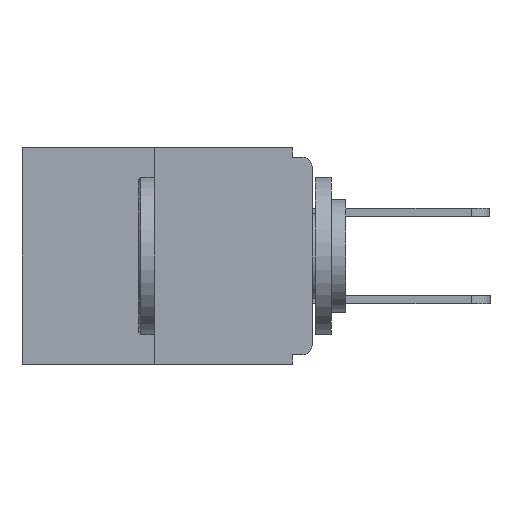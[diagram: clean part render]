
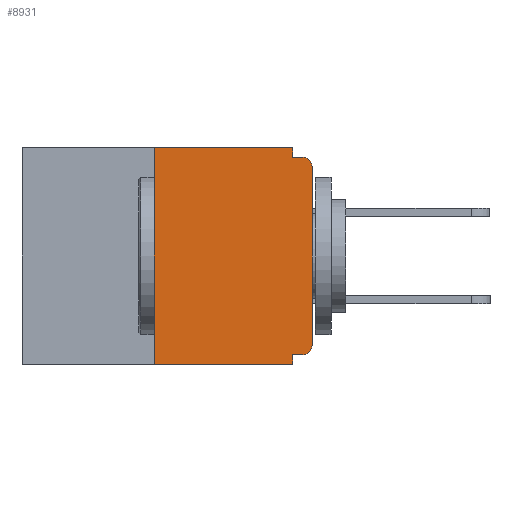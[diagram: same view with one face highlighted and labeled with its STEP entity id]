
A CAD part, left-side view. The second image highlights one B-rep face of the part: STEP entity #8931.
In plain terms, the highlighted planar face has unit normal (-1, 0, 0).
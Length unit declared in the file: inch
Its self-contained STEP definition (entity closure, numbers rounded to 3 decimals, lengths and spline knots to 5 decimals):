
#294 = VECTOR ( 'NONE', #5485, 39.37008 ) ;
#448 = AXIS2_PLACEMENT_3D ( 'NONE', #3779, #9084, #16150 ) ;
#1070 = CARTESIAN_POINT ( 'NONE',  ( 0., 0.031, -0.015 ) ) ;
#1130 = VERTEX_POINT ( 'NONE', #19791 ) ;
#1326 = CARTESIAN_POINT ( 'NONE',  ( 0., 0., -0.328 ) ) ;
#1334 = PLANE ( 'NONE',  #12542 ) ;
#1632 = CARTESIAN_POINT ( 'NONE',  ( 0., 0., -0.015 ) ) ;
#2589 = AXIS2_PLACEMENT_3D ( 'NONE', #32049, #9696, #21960 ) ;
#2727 = EDGE_CURVE ( 'NONE', #11369, #12864, #32143, .T. ) ;
#3448 = VECTOR ( 'NONE', #24528, 39.37008 ) ;
#3747 = LINE ( 'NONE', #1326, #28974 ) ;
#3779 = CARTESIAN_POINT ( 'NONE',  ( 0., 0.015, -0.313 ) ) ;
#4528 = DIRECTION ( 'NONE',  ( 0., 0., 1. ) ) ;
#4813 = LINE ( 'NONE', #25342, #19966 ) ;
#5485 = DIRECTION ( 'NONE',  ( 0., 0., -1. ) ) ;
#5629 = VERTEX_POINT ( 'NONE', #26437 ) ;
#6324 = CARTESIAN_POINT ( 'NONE',  ( 0., 0.46, 0. ) ) ;
#6512 = CARTESIAN_POINT ( 'NONE',  ( 0., 0.25, -0.343 ) ) ;
#6926 = CARTESIAN_POINT ( 'NONE',  ( 0., 0.46, 0. ) ) ;
#7241 = DIRECTION ( 'NONE',  ( 0., 1., 0. ) ) ;
#7750 = EDGE_CURVE ( 'NONE', #29705, #16405, #23504, .T. ) ;
#8355 = LINE ( 'NONE', #27574, #25484 ) ;
#8696 = DIRECTION ( 'NONE',  ( 0., 0., -1. ) ) ;
#8931 = ADVANCED_FACE ( 'NONE', ( #30831 ), #1334, .F. ) ;
#9084 = DIRECTION ( 'NONE',  ( -1., 0., 0. ) ) ;
#9097 = ORIENTED_EDGE ( 'NONE', *, *, #11563, .F. ) ;
#9365 = ORIENTED_EDGE ( 'NONE', *, *, #22293, .F. ) ;
#9696 = DIRECTION ( 'NONE',  ( -1., 0., 0. ) ) ;
#10224 = CARTESIAN_POINT ( 'NONE',  ( 0., 0.46, -0.343 ) ) ;
#10548 = CARTESIAN_POINT ( 'NONE',  ( 0., 0., -0.313 ) ) ;
#11056 = ORIENTED_EDGE ( 'NONE', *, *, #21473, .F. ) ;
#11369 = VERTEX_POINT ( 'NONE', #6512 ) ;
#11563 = EDGE_CURVE ( 'NONE', #15165, #17501, #23261, .T. ) ;
#12345 = VECTOR ( 'NONE', #12535, 39.37008 ) ;
#12535 = DIRECTION ( 'NONE',  ( 0., -1., 0. ) ) ;
#12542 = AXIS2_PLACEMENT_3D ( 'NONE', #6324, #13934, #8696 ) ;
#12823 = LINE ( 'NONE', #22321, #28739 ) ;
#12864 = VERTEX_POINT ( 'NONE', #26837 ) ;
#12969 = EDGE_CURVE ( 'NONE', #17501, #29790, #8355, .T. ) ;
#12984 = ORIENTED_EDGE ( 'NONE', *, *, #2727, .T. ) ;
#13147 = EDGE_LOOP ( 'NONE', ( #9097, #26649, #12984, #11056, #9365, #28401, #31743, #29745, #31501, #24877 ) ) ;
#13517 = CARTESIAN_POINT ( 'NONE',  ( 0., 0.015, -0.015 ) ) ;
#13934 = DIRECTION ( 'NONE',  ( 1., 0., 0. ) ) ;
#14988 = EDGE_CURVE ( 'NONE', #29790, #20738, #15672, .T. ) ;
#15165 = VERTEX_POINT ( 'NONE', #31027 ) ;
#15368 = CARTESIAN_POINT ( 'NONE',  ( 0., 0.031, -0.343 ) ) ;
#15560 = CARTESIAN_POINT ( 'NONE',  ( 0., 0.015, -0.328 ) ) ;
#15672 = LINE ( 'NONE', #1632, #28114 ) ;
#16150 = DIRECTION ( 'NONE',  ( 0., 0., -1. ) ) ;
#16405 = VERTEX_POINT ( 'NONE', #10548 ) ;
#17368 = LINE ( 'NONE', #15368, #294 ) ;
#17501 = VERTEX_POINT ( 'NONE', #20434 ) ;
#19791 = CARTESIAN_POINT ( 'NONE',  ( 0., 0., -0.03 ) ) ;
#19966 = VECTOR ( 'NONE', #25004, 39.37008 ) ;
#20434 = CARTESIAN_POINT ( 'NONE',  ( 0., 0.031, 0. ) ) ;
#20738 = VERTEX_POINT ( 'NONE', #13517 ) ;
#21473 = EDGE_CURVE ( 'NONE', #5629, #12864, #17368, .T. ) ;
#21960 = DIRECTION ( 'NONE',  ( 0., 0., -1. ) ) ;
#22293 = EDGE_CURVE ( 'NONE', #29705, #5629, #3747, .T. ) ;
#22321 = CARTESIAN_POINT ( 'NONE',  ( 0., 0., 0. ) ) ;
#23261 = LINE ( 'NONE', #6926, #3448 ) ;
#23504 = CIRCLE ( 'NONE', #448, 0.015 ) ;
#24528 = DIRECTION ( 'NONE',  ( 0., -1., 0. ) ) ;
#24877 = ORIENTED_EDGE ( 'NONE', *, *, #12969, .F. ) ;
#25004 = DIRECTION ( 'NONE',  ( 0., 0., 1. ) ) ;
#25307 = EDGE_CURVE ( 'NONE', #11369, #15165, #4813, .T. ) ;
#25342 = CARTESIAN_POINT ( 'NONE',  ( 0., 0.25, 0. ) ) ;
#25484 = VECTOR ( 'NONE', #29835, 39.37008 ) ;
#26437 = CARTESIAN_POINT ( 'NONE',  ( 0., 0.031, -0.328 ) ) ;
#26649 = ORIENTED_EDGE ( 'NONE', *, *, #25307, .F. ) ;
#26837 = CARTESIAN_POINT ( 'NONE',  ( 0., 0.031, -0.343 ) ) ;
#27574 = CARTESIAN_POINT ( 'NONE',  ( 0., 0.031, 0. ) ) ;
#27802 = EDGE_CURVE ( 'NONE', #16405, #1130, #12823, .T. ) ;
#28114 = VECTOR ( 'NONE', #28661, 39.37008 ) ;
#28401 = ORIENTED_EDGE ( 'NONE', *, *, #7750, .T. ) ;
#28661 = DIRECTION ( 'NONE',  ( 0., -1., 0. ) ) ;
#28739 = VECTOR ( 'NONE', #4528, 39.37008 ) ;
#28974 = VECTOR ( 'NONE', #7241, 39.37008 ) ;
#29705 = VERTEX_POINT ( 'NONE', #15560 ) ;
#29745 = ORIENTED_EDGE ( 'NONE', *, *, #31049, .T. ) ;
#29790 = VERTEX_POINT ( 'NONE', #1070 ) ;
#29835 = DIRECTION ( 'NONE',  ( 0., 0., -1. ) ) ;
#30283 = CIRCLE ( 'NONE', #2589, 0.015 ) ;
#30831 = FACE_OUTER_BOUND ( 'NONE', #13147, .T. ) ;
#31027 = CARTESIAN_POINT ( 'NONE',  ( 0., 0.25, 0. ) ) ;
#31049 = EDGE_CURVE ( 'NONE', #1130, #20738, #30283, .T. ) ;
#31501 = ORIENTED_EDGE ( 'NONE', *, *, #14988, .F. ) ;
#31743 = ORIENTED_EDGE ( 'NONE', *, *, #27802, .T. ) ;
#32049 = CARTESIAN_POINT ( 'NONE',  ( 0., 0.015, -0.03 ) ) ;
#32143 = LINE ( 'NONE', #10224, #12345 ) ;
